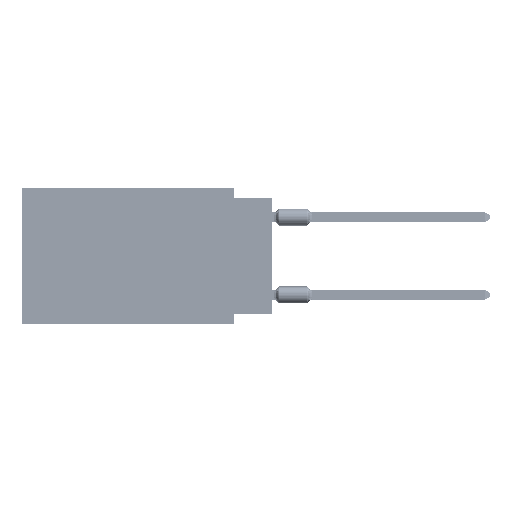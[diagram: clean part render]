
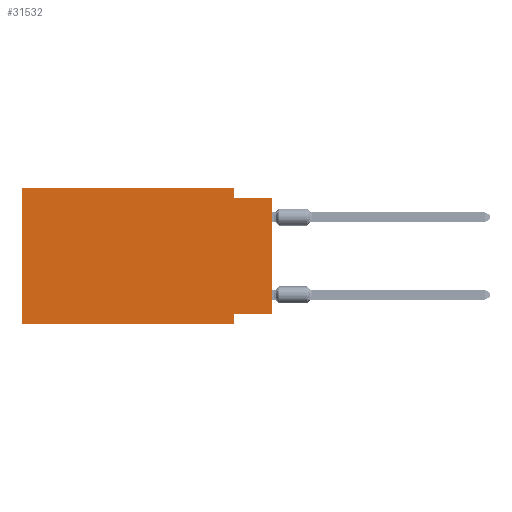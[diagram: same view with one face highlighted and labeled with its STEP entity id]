
A CAD part, left-side view. The second image highlights one B-rep face of the part: STEP entity #31532.
In plain terms, the highlighted planar face has unit normal (-1, 0, 0).
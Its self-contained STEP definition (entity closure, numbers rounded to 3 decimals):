
#1545 = DIRECTION ( 'NONE',  ( 0., 1., 0. ) ) ;
#4468 = CARTESIAN_POINT ( 'NONE',  ( 0., 2.54, 0. ) ) ;
#4513 = VECTOR ( 'NONE', #1545, 1000. ) ;
#5186 = CARTESIAN_POINT ( 'NONE',  ( 0., 16.383, -8.89 ) ) ;
#5473 = ORIENTED_EDGE ( 'NONE', *, *, #18375, .T. ) ;
#5659 = VECTOR ( 'NONE', #19967, 1000. ) ;
#6219 = CARTESIAN_POINT ( 'NONE',  ( 0., 2.54, -8.255 ) ) ;
#9018 = EDGE_LOOP ( 'NONE', ( #26571, #95643, #22727, #13740, #116892, #5473, #103991, #39502 ) ) ;
#11212 = DIRECTION ( 'NONE',  ( 0., 0., -1. ) ) ;
#13740 = ORIENTED_EDGE ( 'NONE', *, *, #113194, .F. ) ;
#18086 = CARTESIAN_POINT ( 'NONE',  ( 0., 2.54, 0. ) ) ;
#18375 = EDGE_CURVE ( 'NONE', #54020, #74072, #98820, .T. ) ;
#18396 = FACE_OUTER_BOUND ( 'NONE', #9018, .T. ) ;
#18404 = LINE ( 'NONE', #83178, #4513 ) ;
#19967 = DIRECTION ( 'NONE',  ( 0., 0., 1. ) ) ;
#22727 = ORIENTED_EDGE ( 'NONE', *, *, #78279, .F. ) ;
#26571 = ORIENTED_EDGE ( 'NONE', *, *, #95556, .T. ) ;
#27392 = DIRECTION ( 'NONE',  ( 1., 0., 0. ) ) ;
#27979 = CARTESIAN_POINT ( 'NONE',  ( 0., 0., -8.255 ) ) ;
#29654 = VECTOR ( 'NONE', #79035, 1000. ) ;
#31532 = ADVANCED_FACE ( 'NONE', ( #18396 ), #36383, .F. ) ;
#31661 = CARTESIAN_POINT ( 'NONE',  ( 0., 0., -0.635 ) ) ;
#36383 = PLANE ( 'NONE',  #57253 ) ;
#36592 = EDGE_CURVE ( 'NONE', #73298, #117024, #18404, .T. ) ;
#38131 = VECTOR ( 'NONE', #50445, 1000. ) ;
#39502 = ORIENTED_EDGE ( 'NONE', *, *, #36592, .F. ) ;
#41732 = LINE ( 'NONE', #115565, #71035 ) ;
#42652 = CARTESIAN_POINT ( 'NONE',  ( 0., 0., -0.635 ) ) ;
#45383 = DIRECTION ( 'NONE',  ( 0., 0., -1. ) ) ;
#48083 = CARTESIAN_POINT ( 'NONE',  ( 0., 16.383, 0. ) ) ;
#50445 = DIRECTION ( 'NONE',  ( 0., -1., 0. ) ) ;
#53481 = LINE ( 'NONE', #99728, #58794 ) ;
#54020 = VERTEX_POINT ( 'NONE', #5186 ) ;
#55351 = LINE ( 'NONE', #100419, #5659 ) ;
#57253 = AXIS2_PLACEMENT_3D ( 'NONE', #116839, #27392, #45383 ) ;
#58794 = VECTOR ( 'NONE', #100321, 1000. ) ;
#63666 = DIRECTION ( 'NONE',  ( 0., 0., -1. ) ) ;
#64638 = VERTEX_POINT ( 'NONE', #73809 ) ;
#65797 = CARTESIAN_POINT ( 'NONE',  ( 0., 2.54, -8.89 ) ) ;
#69320 = EDGE_CURVE ( 'NONE', #54020, #93278, #55351, .T. ) ;
#69434 = CARTESIAN_POINT ( 'NONE',  ( 0., 16.383, -8.89 ) ) ;
#71035 = VECTOR ( 'NONE', #88545, 1000. ) ;
#72065 = LINE ( 'NONE', #18086, #87376 ) ;
#73043 = VERTEX_POINT ( 'NONE', #4468 ) ;
#73298 = VERTEX_POINT ( 'NONE', #27979 ) ;
#73809 = CARTESIAN_POINT ( 'NONE',  ( 0., 2.54, -0.635 ) ) ;
#74072 = VERTEX_POINT ( 'NONE', #82904 ) ;
#78279 = EDGE_CURVE ( 'NONE', #73043, #64638, #72065, .T. ) ;
#79035 = DIRECTION ( 'NONE',  ( 0., -1., 0. ) ) ;
#82904 = CARTESIAN_POINT ( 'NONE',  ( 0., 2.54, -8.89 ) ) ;
#83178 = CARTESIAN_POINT ( 'NONE',  ( 0., 0., -8.255 ) ) ;
#87376 = VECTOR ( 'NONE', #63666, 1000. ) ;
#88545 = DIRECTION ( 'NONE',  ( 0., 0., 1. ) ) ;
#93278 = VERTEX_POINT ( 'NONE', #48083 ) ;
#93412 = LINE ( 'NONE', #65797, #101484 ) ;
#93464 = EDGE_CURVE ( 'NONE', #64638, #103506, #96087, .T. ) ;
#95556 = EDGE_CURVE ( 'NONE', #73298, #103506, #41732, .T. ) ;
#95643 = ORIENTED_EDGE ( 'NONE', *, *, #93464, .F. ) ;
#96087 = LINE ( 'NONE', #42652, #38131 ) ;
#98820 = LINE ( 'NONE', #69434, #29654 ) ;
#99728 = CARTESIAN_POINT ( 'NONE',  ( 0., 16.383, 0. ) ) ;
#100321 = DIRECTION ( 'NONE',  ( 0., -1., 0. ) ) ;
#100419 = CARTESIAN_POINT ( 'NONE',  ( 0., 16.383, 0. ) ) ;
#101484 = VECTOR ( 'NONE', #11212, 1000. ) ;
#103506 = VERTEX_POINT ( 'NONE', #31661 ) ;
#103991 = ORIENTED_EDGE ( 'NONE', *, *, #116318, .F. ) ;
#113194 = EDGE_CURVE ( 'NONE', #93278, #73043, #53481, .T. ) ;
#115565 = CARTESIAN_POINT ( 'NONE',  ( 0., 0., 0. ) ) ;
#116318 = EDGE_CURVE ( 'NONE', #117024, #74072, #93412, .T. ) ;
#116839 = CARTESIAN_POINT ( 'NONE',  ( 0., 16.383, 0. ) ) ;
#116892 = ORIENTED_EDGE ( 'NONE', *, *, #69320, .F. ) ;
#117024 = VERTEX_POINT ( 'NONE', #6219 ) ;
